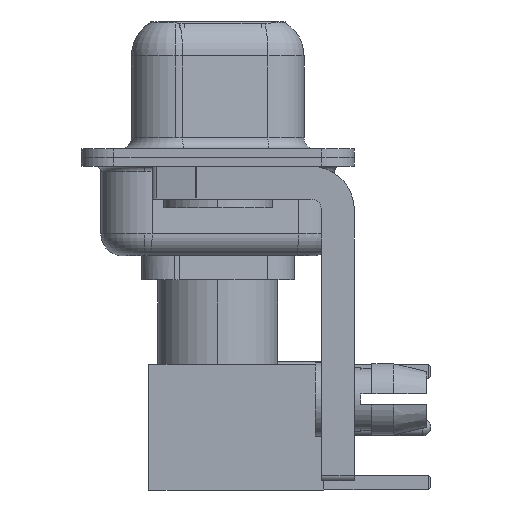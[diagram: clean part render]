
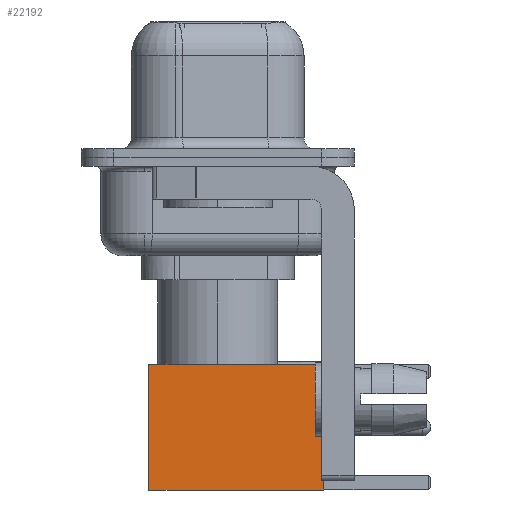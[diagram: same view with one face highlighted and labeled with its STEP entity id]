
A CAD part, left-side view. The second image highlights one B-rep face of the part: STEP entity #22192.
In plain terms, the highlighted face is planar.
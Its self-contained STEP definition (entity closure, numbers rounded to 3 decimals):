
#197 = VERTEX_POINT ( 'NONE', #5627 ) ;
#2692 = LINE ( 'NONE', #24917, #26027 ) ;
#2705 = CARTESIAN_POINT ( 'NONE',  ( 2.875, 2.875, 0. ) ) ;
#3410 = EDGE_CURVE ( 'NONE', #25684, #22162, #10776, .T. ) ;
#3415 = EDGE_CURVE ( 'NONE', #27799, #22162, #8194, .T. ) ;
#4571 = VECTOR ( 'NONE', #25572, 1000. ) ;
#5627 = CARTESIAN_POINT ( 'NONE',  ( 2.875, 2.875, 8. ) ) ;
#8194 = LINE ( 'NONE', #16972, #4571 ) ;
#8340 = ORIENTED_EDGE ( 'NONE', *, *, #3410, .F. ) ;
#8445 = CARTESIAN_POINT ( 'NONE',  ( 2.875, 2.875, 0. ) ) ;
#8733 = PLANE ( 'NONE',  #9033 ) ;
#9014 = CARTESIAN_POINT ( 'NONE',  ( -2.875, 2.875, 0. ) ) ;
#9033 = AXIS2_PLACEMENT_3D ( 'NONE', #8445, #17648, #19665 ) ;
#10288 = ORIENTED_EDGE ( 'NONE', *, *, #11324, .T. ) ;
#10776 = LINE ( 'NONE', #19403, #14653 ) ;
#11324 = EDGE_CURVE ( 'NONE', #197, #27799, #15756, .T. ) ;
#13907 = ORIENTED_EDGE ( 'NONE', *, *, #24270, .F. ) ;
#14653 = VECTOR ( 'NONE', #25857, 1000. ) ;
#15371 = ORIENTED_EDGE ( 'NONE', *, *, #3415, .T. ) ;
#15756 = LINE ( 'NONE', #2705, #17801 ) ;
#16972 = CARTESIAN_POINT ( 'NONE',  ( 0., 2.875, 0. ) ) ;
#17648 = DIRECTION ( 'NONE',  ( 0., 1., 0. ) ) ;
#17801 = VECTOR ( 'NONE', #20203, 1000. ) ;
#18333 = CARTESIAN_POINT ( 'NONE',  ( -2.875, 2.875, 8. ) ) ;
#19403 = CARTESIAN_POINT ( 'NONE',  ( -2.875, 2.875, 0. ) ) ;
#19665 = DIRECTION ( 'NONE',  ( 0., 0., 1. ) ) ;
#20203 = DIRECTION ( 'NONE',  ( 0., 0., -1. ) ) ;
#21584 = CARTESIAN_POINT ( 'NONE',  ( 2.875, 2.875, 0. ) ) ;
#22162 = VERTEX_POINT ( 'NONE', #9014 ) ;
#22192 = ADVANCED_FACE ( 'NONE', ( #23814 ), #8733, .T. ) ;
#23814 = FACE_OUTER_BOUND ( 'NONE', #27459, .T. ) ;
#24270 = EDGE_CURVE ( 'NONE', #197, #25684, #2692, .T. ) ;
#24628 = DIRECTION ( 'NONE',  ( -1., 0., 0. ) ) ;
#24917 = CARTESIAN_POINT ( 'NONE',  ( 0., 2.875, 8. ) ) ;
#25572 = DIRECTION ( 'NONE',  ( -1., 0., 0. ) ) ;
#25684 = VERTEX_POINT ( 'NONE', #18333 ) ;
#25857 = DIRECTION ( 'NONE',  ( 0., 0., -1. ) ) ;
#26027 = VECTOR ( 'NONE', #24628, 1000. ) ;
#27459 = EDGE_LOOP ( 'NONE', ( #10288, #15371, #8340, #13907 ) ) ;
#27799 = VERTEX_POINT ( 'NONE', #21584 ) ;
